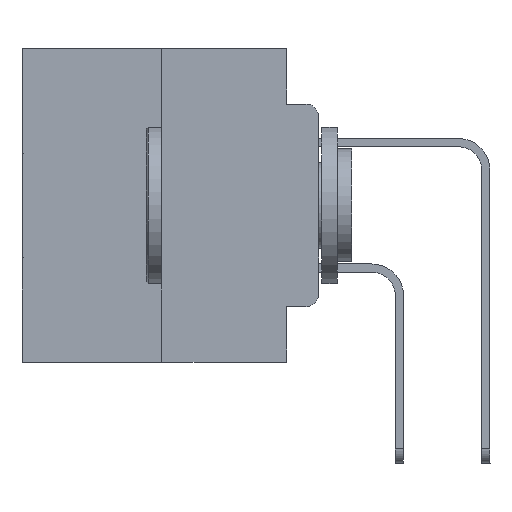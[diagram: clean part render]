
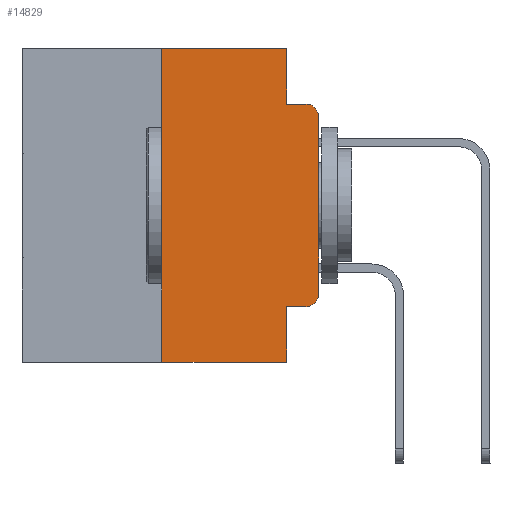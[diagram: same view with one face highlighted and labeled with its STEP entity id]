
A CAD part, left-side view. The second image highlights one B-rep face of the part: STEP entity #14829.
In plain terms, the highlighted planar face has unit normal (-1, 0, 0).
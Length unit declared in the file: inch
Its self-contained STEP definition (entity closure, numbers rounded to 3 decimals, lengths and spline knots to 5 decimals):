
#588 = AXIS2_PLACEMENT_3D ( 'NONE', #4135, #20110, #6537 ) ;
#1616 = CARTESIAN_POINT ( 'NONE',  ( 0., 0.25, -0.5 ) ) ;
#2537 = VERTEX_POINT ( 'NONE', #1616 ) ;
#2728 = AXIS2_PLACEMENT_3D ( 'NONE', #12953, #28423, #15209 ) ;
#2747 = DIRECTION ( 'NONE',  ( 0., -1., 0. ) ) ;
#2896 = DIRECTION ( 'NONE',  ( 0., -1., 0. ) ) ;
#3063 = EDGE_CURVE ( 'NONE', #21222, #14099, #21795, .T. ) ;
#3291 = ORIENTED_EDGE ( 'NONE', *, *, #7126, .F. ) ;
#3614 = VECTOR ( 'NONE', #7321, 39.37008 ) ;
#3880 = CARTESIAN_POINT ( 'NONE',  ( 0., 0.051, -0.0885 ) ) ;
#3987 = FACE_OUTER_BOUND ( 'NONE', #21809, .T. ) ;
#4135 = CARTESIAN_POINT ( 'NONE',  ( 0., 0.02, -0.1085 ) ) ;
#4694 = EDGE_CURVE ( 'NONE', #21222, #27210, #17601, .T. ) ;
#4749 = CARTESIAN_POINT ( 'NONE',  ( 0., 0.25, 0. ) ) ;
#4872 = VERTEX_POINT ( 'NONE', #4749 ) ;
#6197 = CARTESIAN_POINT ( 'NONE',  ( 0., 0.051, -0.5 ) ) ;
#6388 = LINE ( 'NONE', #3880, #10697 ) ;
#6536 = EDGE_CURVE ( 'NONE', #24751, #26068, #18895, .T. ) ;
#6537 = DIRECTION ( 'NONE',  ( 0., 0., -1. ) ) ;
#6640 = CARTESIAN_POINT ( 'NONE',  ( 0., 0.051, 0. ) ) ;
#7053 = CARTESIAN_POINT ( 'NONE',  ( 0., 0., 0. ) ) ;
#7065 = ORIENTED_EDGE ( 'NONE', *, *, #3063, .T. ) ;
#7126 = EDGE_CURVE ( 'NONE', #24443, #26068, #6388, .T. ) ;
#7214 = VECTOR ( 'NONE', #2896, 39.37008 ) ;
#7321 = DIRECTION ( 'NONE',  ( 0., -1., 0. ) ) ;
#7404 = VERTEX_POINT ( 'NONE', #16412 ) ;
#7880 = CIRCLE ( 'NONE', #2728, 0.02 ) ;
#8375 = CARTESIAN_POINT ( 'NONE',  ( 0., 0.02, -0.4115 ) ) ;
#8386 = CARTESIAN_POINT ( 'NONE',  ( 0., 0., -0.1085 ) ) ;
#8713 = CARTESIAN_POINT ( 'NONE',  ( 0., 0.051, -0.4115 ) ) ;
#9199 = VERTEX_POINT ( 'NONE', #11700 ) ;
#10335 = ORIENTED_EDGE ( 'NONE', *, *, #21436, .F. ) ;
#10697 = VECTOR ( 'NONE', #24273, 39.37008 ) ;
#11582 = VECTOR ( 'NONE', #22783, 39.37008 ) ;
#11700 = CARTESIAN_POINT ( 'NONE',  ( 0., 0.051, 0. ) ) ;
#12953 = CARTESIAN_POINT ( 'NONE',  ( 0., 0.02, -0.3915 ) ) ;
#13158 = DIRECTION ( 'NONE',  ( 0., 0., -1. ) ) ;
#13345 = LINE ( 'NONE', #21111, #7214 ) ;
#14046 = EDGE_CURVE ( 'NONE', #2537, #4872, #14242, .T. ) ;
#14099 = VERTEX_POINT ( 'NONE', #8375 ) ;
#14242 = LINE ( 'NONE', #21545, #25267 ) ;
#14739 = CARTESIAN_POINT ( 'NONE',  ( 0., 0.051, -0.4115 ) ) ;
#14829 = ADVANCED_FACE ( 'NONE', ( #3987 ), #21982, .F. ) ;
#15209 = DIRECTION ( 'NONE',  ( 0., 0., -1. ) ) ;
#16412 = CARTESIAN_POINT ( 'NONE',  ( 0., 0., -0.3915 ) ) ;
#16892 = LINE ( 'NONE', #7053, #11582 ) ;
#17256 = EDGE_CURVE ( 'NONE', #7404, #24751, #16892, .T. ) ;
#17338 = LINE ( 'NONE', #23166, #27639 ) ;
#17422 = CARTESIAN_POINT ( 'NONE',  ( 0., 0.051, -0.0885 ) ) ;
#17535 = LINE ( 'NONE', #17743, #22672 ) ;
#17601 = LINE ( 'NONE', #6640, #29329 ) ;
#17743 = CARTESIAN_POINT ( 'NONE',  ( 0., 0.051, 0. ) ) ;
#17762 = CARTESIAN_POINT ( 'NONE',  ( 0., 0.02, -0.0885 ) ) ;
#18450 = ORIENTED_EDGE ( 'NONE', *, *, #4694, .F. ) ;
#18895 = CIRCLE ( 'NONE', #588, 0.02 ) ;
#20110 = DIRECTION ( 'NONE',  ( -1., 0., 0. ) ) ;
#20206 = DIRECTION ( 'NONE',  ( 0., 0., -1. ) ) ;
#20851 = ORIENTED_EDGE ( 'NONE', *, *, #6536, .T. ) ;
#21111 = CARTESIAN_POINT ( 'NONE',  ( 0., 0.473, -0.5 ) ) ;
#21159 = EDGE_CURVE ( 'NONE', #2537, #27210, #13345, .T. ) ;
#21222 = VERTEX_POINT ( 'NONE', #14739 ) ;
#21436 = EDGE_CURVE ( 'NONE', #9199, #24443, #17535, .T. ) ;
#21545 = CARTESIAN_POINT ( 'NONE',  ( 0., 0.25, 0. ) ) ;
#21555 = AXIS2_PLACEMENT_3D ( 'NONE', #26290, #26387, #13158 ) ;
#21795 = LINE ( 'NONE', #8713, #3614 ) ;
#21809 = EDGE_LOOP ( 'NONE', ( #25286, #20851, #3291, #10335, #22208, #22896, #28759, #18450, #7065, #27031 ) ) ;
#21982 = PLANE ( 'NONE',  #21555 ) ;
#21984 = EDGE_CURVE ( 'NONE', #14099, #7404, #7880, .T. ) ;
#22138 = DIRECTION ( 'NONE',  ( 0., 0., -1. ) ) ;
#22208 = ORIENTED_EDGE ( 'NONE', *, *, #26917, .F. ) ;
#22672 = VECTOR ( 'NONE', #22138, 39.37008 ) ;
#22783 = DIRECTION ( 'NONE',  ( 0., 0., 1. ) ) ;
#22896 = ORIENTED_EDGE ( 'NONE', *, *, #14046, .F. ) ;
#23166 = CARTESIAN_POINT ( 'NONE',  ( 0., 0.473, 0. ) ) ;
#23733 = DIRECTION ( 'NONE',  ( 0., 0., 1. ) ) ;
#24273 = DIRECTION ( 'NONE',  ( 0., -1., 0. ) ) ;
#24443 = VERTEX_POINT ( 'NONE', #17422 ) ;
#24751 = VERTEX_POINT ( 'NONE', #8386 ) ;
#25267 = VECTOR ( 'NONE', #23733, 39.37008 ) ;
#25286 = ORIENTED_EDGE ( 'NONE', *, *, #17256, .T. ) ;
#26068 = VERTEX_POINT ( 'NONE', #17762 ) ;
#26290 = CARTESIAN_POINT ( 'NONE',  ( 0., 0.473, 0. ) ) ;
#26387 = DIRECTION ( 'NONE',  ( 1., 0., 0. ) ) ;
#26917 = EDGE_CURVE ( 'NONE', #4872, #9199, #17338, .T. ) ;
#27031 = ORIENTED_EDGE ( 'NONE', *, *, #21984, .T. ) ;
#27210 = VERTEX_POINT ( 'NONE', #6197 ) ;
#27639 = VECTOR ( 'NONE', #2747, 39.37008 ) ;
#28423 = DIRECTION ( 'NONE',  ( -1., 0., 0. ) ) ;
#28759 = ORIENTED_EDGE ( 'NONE', *, *, #21159, .T. ) ;
#29329 = VECTOR ( 'NONE', #20206, 39.37008 ) ;
